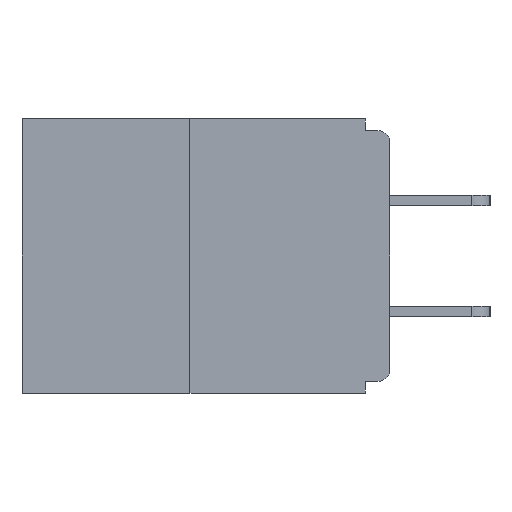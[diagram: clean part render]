
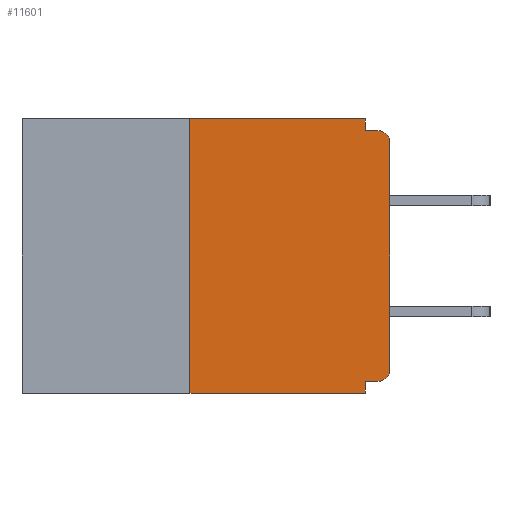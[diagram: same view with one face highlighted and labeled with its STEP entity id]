
A CAD part, left-side view. The second image highlights one B-rep face of the part: STEP entity #11601.
In plain terms, the highlighted planar face has unit normal (-1, 0, 0).
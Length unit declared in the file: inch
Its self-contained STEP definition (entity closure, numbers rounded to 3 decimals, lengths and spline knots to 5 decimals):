
#73 = LINE ( 'NONE', #11270, #7880 ) ;
#178 = FACE_OUTER_BOUND ( 'NONE', #4159, .T. ) ;
#200 = VECTOR ( 'NONE', #2709, 39.37008 ) ;
#205 = ORIENTED_EDGE ( 'NONE', *, *, #3678, .T. ) ;
#381 = VERTEX_POINT ( 'NONE', #10823 ) ;
#407 = DIRECTION ( 'NONE',  ( -1., 0., 0. ) ) ;
#484 = CARTESIAN_POINT ( 'NONE',  ( 0., 0.015, -0.015 ) ) ;
#600 = ORIENTED_EDGE ( 'NONE', *, *, #15194, .T. ) ;
#637 = ORIENTED_EDGE ( 'NONE', *, *, #15219, .F. ) ;
#676 = LINE ( 'NONE', #10574, #4838 ) ;
#1148 = VERTEX_POINT ( 'NONE', #2983 ) ;
#1256 = ORIENTED_EDGE ( 'NONE', *, *, #6299, .F. ) ;
#1946 = AXIS2_PLACEMENT_3D ( 'NONE', #6241, #7386, #3717 ) ;
#2709 = DIRECTION ( 'NONE',  ( 0., -1., 0. ) ) ;
#2983 = CARTESIAN_POINT ( 'NONE',  ( 0., 0., -0.313 ) ) ;
#3146 = EDGE_CURVE ( 'NONE', #13218, #13791, #10413, .T. ) ;
#3151 = CARTESIAN_POINT ( 'NONE',  ( 0., 0.031, 0. ) ) ;
#3170 = DIRECTION ( 'NONE',  ( 0., 0., -1. ) ) ;
#3528 = VECTOR ( 'NONE', #9751, 39.37008 ) ;
#3544 = AXIS2_PLACEMENT_3D ( 'NONE', #12814, #407, #3802 ) ;
#3678 = EDGE_CURVE ( 'NONE', #8931, #13791, #5889, .T. ) ;
#3717 = DIRECTION ( 'NONE',  ( 0., 0., -1. ) ) ;
#3802 = DIRECTION ( 'NONE',  ( 0., 0., -1. ) ) ;
#3890 = DIRECTION ( 'NONE',  ( 0., 0., 1. ) ) ;
#4159 = EDGE_LOOP ( 'NONE', ( #10322, #1256, #600, #637, #15865, #14127, #12742, #205, #12901, #5271 ) ) ;
#4565 = CARTESIAN_POINT ( 'NONE',  ( 0., 0.015, -0.313 ) ) ;
#4838 = VECTOR ( 'NONE', #10486, 39.37008 ) ;
#5271 = ORIENTED_EDGE ( 'NONE', *, *, #12520, .F. ) ;
#5375 = VECTOR ( 'NONE', #3890, 39.37008 ) ;
#5889 = CIRCLE ( 'NONE', #3544, 0.015 ) ;
#6204 = AXIS2_PLACEMENT_3D ( 'NONE', #4565, #15987, #8542 ) ;
#6241 = CARTESIAN_POINT ( 'NONE',  ( 0., 0.46, 0. ) ) ;
#6255 = CARTESIAN_POINT ( 'NONE',  ( 0., 0., -0.328 ) ) ;
#6299 = EDGE_CURVE ( 'NONE', #12587, #381, #8600, .T. ) ;
#6882 = VERTEX_POINT ( 'NONE', #3151 ) ;
#7386 = DIRECTION ( 'NONE',  ( 1., 0., 0. ) ) ;
#7776 = CIRCLE ( 'NONE', #6204, 0.015 ) ;
#7880 = VECTOR ( 'NONE', #13685, 39.37008 ) ;
#8091 = CARTESIAN_POINT ( 'NONE',  ( 0., 0.015, -0.328 ) ) ;
#8542 = DIRECTION ( 'NONE',  ( 0., 0., -1. ) ) ;
#8600 = LINE ( 'NONE', #8765, #5375 ) ;
#8765 = CARTESIAN_POINT ( 'NONE',  ( 0., 0.25, 0. ) ) ;
#8931 = VERTEX_POINT ( 'NONE', #10933 ) ;
#8948 = CARTESIAN_POINT ( 'NONE',  ( 0., 0.031, -0.343 ) ) ;
#9240 = LINE ( 'NONE', #12723, #10984 ) ;
#9751 = DIRECTION ( 'NONE',  ( 0., 1., 0. ) ) ;
#9905 = PLANE ( 'NONE',  #1946 ) ;
#10022 = VERTEX_POINT ( 'NONE', #8948 ) ;
#10322 = ORIENTED_EDGE ( 'NONE', *, *, #14620, .F. ) ;
#10413 = LINE ( 'NONE', #12684, #11080 ) ;
#10486 = DIRECTION ( 'NONE',  ( 0., -1., 0. ) ) ;
#10574 = CARTESIAN_POINT ( 'NONE',  ( 0., 0.46, -0.343 ) ) ;
#10823 = CARTESIAN_POINT ( 'NONE',  ( 0., 0.25, 0. ) ) ;
#10933 = CARTESIAN_POINT ( 'NONE',  ( 0., 0., -0.03 ) ) ;
#10973 = LINE ( 'NONE', #6255, #3528 ) ;
#10984 = VECTOR ( 'NONE', #14092, 39.37008 ) ;
#11063 = EDGE_CURVE ( 'NONE', #14377, #1148, #7776, .T. ) ;
#11080 = VECTOR ( 'NONE', #12760, 39.37008 ) ;
#11270 = CARTESIAN_POINT ( 'NONE',  ( 0., 0., 0. ) ) ;
#11600 = CARTESIAN_POINT ( 'NONE',  ( 0., 0.031, -0.328 ) ) ;
#11601 = ADVANCED_FACE ( 'NONE', ( #178 ), #9905, .F. ) ;
#12035 = EDGE_CURVE ( 'NONE', #1148, #8931, #73, .T. ) ;
#12383 = VECTOR ( 'NONE', #3170, 39.37008 ) ;
#12520 = EDGE_CURVE ( 'NONE', #6882, #13218, #9240, .T. ) ;
#12587 = VERTEX_POINT ( 'NONE', #14014 ) ;
#12589 = VERTEX_POINT ( 'NONE', #11600 ) ;
#12684 = CARTESIAN_POINT ( 'NONE',  ( 0., 0., -0.015 ) ) ;
#12723 = CARTESIAN_POINT ( 'NONE',  ( 0., 0.031, 0. ) ) ;
#12742 = ORIENTED_EDGE ( 'NONE', *, *, #12035, .T. ) ;
#12760 = DIRECTION ( 'NONE',  ( 0., -1., 0. ) ) ;
#12814 = CARTESIAN_POINT ( 'NONE',  ( 0., 0.015, -0.03 ) ) ;
#12901 = ORIENTED_EDGE ( 'NONE', *, *, #3146, .F. ) ;
#13218 = VERTEX_POINT ( 'NONE', #15914 ) ;
#13685 = DIRECTION ( 'NONE',  ( 0., 0., 1. ) ) ;
#13791 = VERTEX_POINT ( 'NONE', #484 ) ;
#14014 = CARTESIAN_POINT ( 'NONE',  ( 0., 0.25, -0.343 ) ) ;
#14092 = DIRECTION ( 'NONE',  ( 0., 0., -1. ) ) ;
#14127 = ORIENTED_EDGE ( 'NONE', *, *, #11063, .T. ) ;
#14286 = CARTESIAN_POINT ( 'NONE',  ( 0., 0.031, -0.343 ) ) ;
#14377 = VERTEX_POINT ( 'NONE', #8091 ) ;
#14445 = LINE ( 'NONE', #14286, #12383 ) ;
#14620 = EDGE_CURVE ( 'NONE', #381, #6882, #15356, .T. ) ;
#14884 = EDGE_CURVE ( 'NONE', #14377, #12589, #10973, .T. ) ;
#15194 = EDGE_CURVE ( 'NONE', #12587, #10022, #676, .T. ) ;
#15205 = CARTESIAN_POINT ( 'NONE',  ( 0., 0.46, 0. ) ) ;
#15219 = EDGE_CURVE ( 'NONE', #12589, #10022, #14445, .T. ) ;
#15356 = LINE ( 'NONE', #15205, #200 ) ;
#15865 = ORIENTED_EDGE ( 'NONE', *, *, #14884, .F. ) ;
#15914 = CARTESIAN_POINT ( 'NONE',  ( 0., 0.031, -0.015 ) ) ;
#15987 = DIRECTION ( 'NONE',  ( -1., 0., 0. ) ) ;
